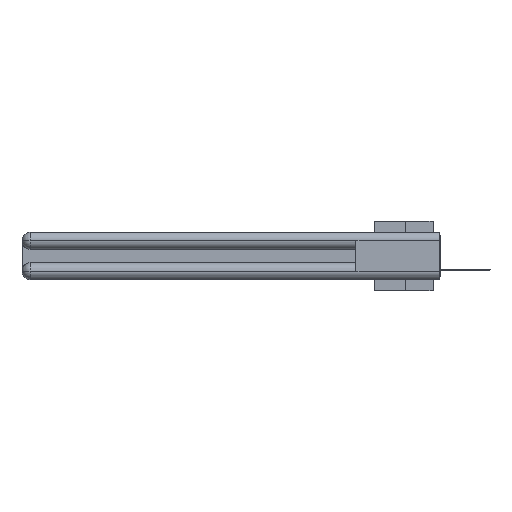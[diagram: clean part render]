
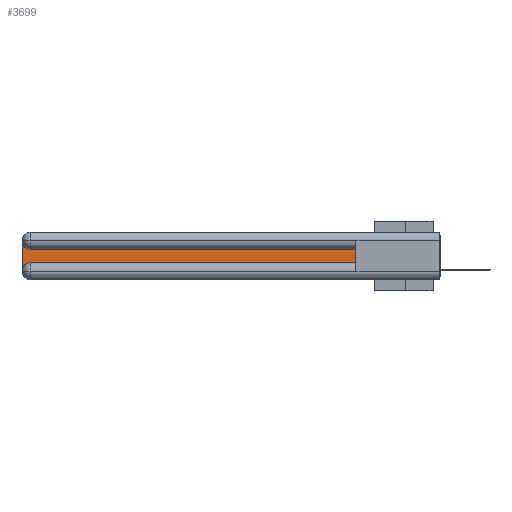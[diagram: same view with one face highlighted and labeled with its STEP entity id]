
A CAD part, left-side view. The second image highlights one B-rep face of the part: STEP entity #3699.
In plain terms, the highlighted planar face has unit normal (-1, 0, 0).
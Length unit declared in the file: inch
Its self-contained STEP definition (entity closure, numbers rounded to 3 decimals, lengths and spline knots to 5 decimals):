
#239 = VECTOR ( 'NONE', #2389, 39.37008 ) ;
#2389 = DIRECTION ( 'NONE',  ( 0., 0., -1. ) ) ;
#2485 = CARTESIAN_POINT ( 'NONE',  ( 0.075, 0.6, -0.2175 ) ) ;
#2754 = ORIENTED_EDGE ( 'NONE', *, *, #29146, .T. ) ;
#3030 = LINE ( 'NONE', #31501, #30452 ) ;
#3066 = ORIENTED_EDGE ( 'NONE', *, *, #18657, .T. ) ;
#3699 = ADVANCED_FACE ( 'NONE', ( #22620 ), #17527, .F. ) ;
#4476 = CARTESIAN_POINT ( 'NONE',  ( 0.075, 0.6, -0.1225 ) ) ;
#4881 = EDGE_CURVE ( 'NONE', #28729, #10439, #22132, .T. ) ;
#5638 = ORIENTED_EDGE ( 'NONE', *, *, #4881, .T. ) ;
#5639 = VERTEX_POINT ( 'NONE', #13337 ) ;
#6575 = CIRCLE ( 'NONE', #19572, 0.06 ) ;
#6672 = EDGE_CURVE ( 'NONE', #7035, #29035, #33317, .T. ) ;
#7035 = VERTEX_POINT ( 'NONE', #30249 ) ;
#7311 = CARTESIAN_POINT ( 'NONE',  ( 0.075, 3., -0.2175 ) ) ;
#8288 = DIRECTION ( 'NONE',  ( 0., 0., 1. ) ) ;
#8832 = DIRECTION ( 'NONE',  ( 0., 0., -1. ) ) ;
#8858 = EDGE_CURVE ( 'NONE', #19188, #7035, #21831, .T. ) ;
#9263 = CARTESIAN_POINT ( 'NONE',  ( 0.075, 2.94, -0.0625 ) ) ;
#9700 = CARTESIAN_POINT ( 'NONE',  ( 0.075, 0.6, -0.2175 ) ) ;
#10439 = VERTEX_POINT ( 'NONE', #15422 ) ;
#13337 = CARTESIAN_POINT ( 'NONE',  ( 0.075, 3., -0.0625 ) ) ;
#14159 = VECTOR ( 'NONE', #31111, 39.37008 ) ;
#14265 = DIRECTION ( 'NONE',  ( 1., 0., 0. ) ) ;
#14596 = CARTESIAN_POINT ( 'NONE',  ( 0.075, 2.94, -0.2775 ) ) ;
#14996 = CARTESIAN_POINT ( 'NONE',  ( 0.075, 3., -0.1225 ) ) ;
#15316 = DIRECTION ( 'NONE',  ( 1., 0., 0. ) ) ;
#15422 = CARTESIAN_POINT ( 'NONE',  ( 0.075, 2.94, -0.1225 ) ) ;
#15466 = DIRECTION ( 'NONE',  ( 0., 0., -1. ) ) ;
#16293 = VECTOR ( 'NONE', #27542, 39.37008 ) ;
#17527 = PLANE ( 'NONE',  #28122 ) ;
#18020 = EDGE_CURVE ( 'NONE', #29035, #28729, #3030, .T. ) ;
#18657 = EDGE_CURVE ( 'NONE', #10439, #5639, #6575, .T. ) ;
#19188 = VERTEX_POINT ( 'NONE', #30331 ) ;
#19320 = EDGE_LOOP ( 'NONE', ( #5638, #3066, #2754, #26318, #25296, #29695 ) ) ;
#19572 = AXIS2_PLACEMENT_3D ( 'NONE', #9263, #31039, #15466 ) ;
#20225 = DIRECTION ( 'NONE',  ( 0., 0., -1. ) ) ;
#21831 = CIRCLE ( 'NONE', #26161, 0.06 ) ;
#22132 = LINE ( 'NONE', #4476, #16293 ) ;
#22620 = FACE_OUTER_BOUND ( 'NONE', #19320, .T. ) ;
#25296 = ORIENTED_EDGE ( 'NONE', *, *, #6672, .T. ) ;
#25599 = LINE ( 'NONE', #7311, #239 ) ;
#26161 = AXIS2_PLACEMENT_3D ( 'NONE', #14596, #14265, #8832 ) ;
#26318 = ORIENTED_EDGE ( 'NONE', *, *, #8858, .T. ) ;
#27542 = DIRECTION ( 'NONE',  ( 0., 1., 0. ) ) ;
#28026 = CARTESIAN_POINT ( 'NONE',  ( 0.075, 0.6, -0.1225 ) ) ;
#28122 = AXIS2_PLACEMENT_3D ( 'NONE', #14996, #15316, #20225 ) ;
#28729 = VERTEX_POINT ( 'NONE', #28026 ) ;
#29035 = VERTEX_POINT ( 'NONE', #9700 ) ;
#29146 = EDGE_CURVE ( 'NONE', #5639, #19188, #25599, .T. ) ;
#29695 = ORIENTED_EDGE ( 'NONE', *, *, #18020, .T. ) ;
#30249 = CARTESIAN_POINT ( 'NONE',  ( 0.075, 2.94, -0.2175 ) ) ;
#30331 = CARTESIAN_POINT ( 'NONE',  ( 0.075, 3., -0.2775 ) ) ;
#30452 = VECTOR ( 'NONE', #8288, 39.37008 ) ;
#31039 = DIRECTION ( 'NONE',  ( 1., 0., 0. ) ) ;
#31111 = DIRECTION ( 'NONE',  ( 0., -1., 0. ) ) ;
#31501 = CARTESIAN_POINT ( 'NONE',  ( 0.075, 0.6, -0.2175 ) ) ;
#33317 = LINE ( 'NONE', #2485, #14159 ) ;
